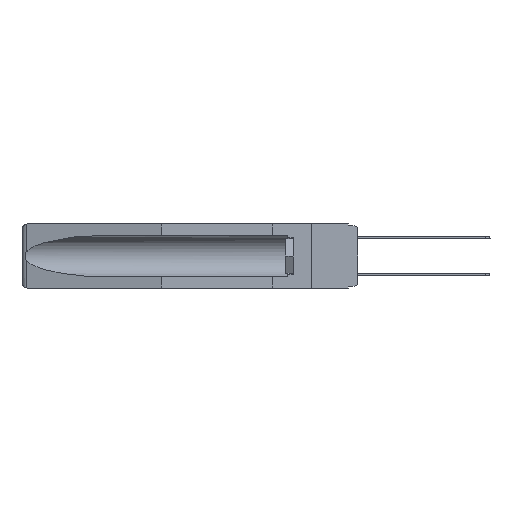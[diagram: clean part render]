
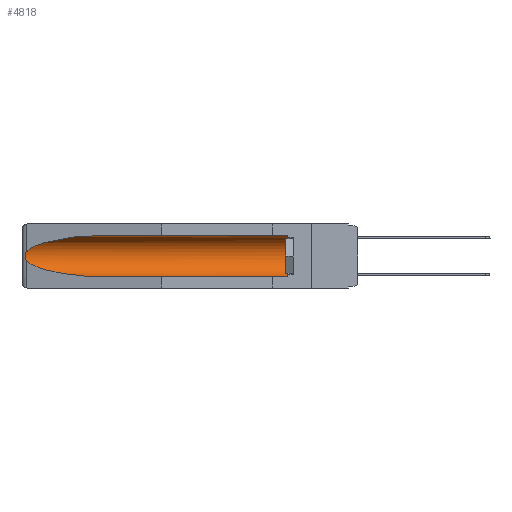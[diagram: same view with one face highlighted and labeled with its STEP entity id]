
A CAD part, left-side view. The second image highlights one B-rep face of the part: STEP entity #4818.
In plain terms, the highlighted cylindrical face has radius 2.857 mm (diameter 5.715 mm), a partial arc.
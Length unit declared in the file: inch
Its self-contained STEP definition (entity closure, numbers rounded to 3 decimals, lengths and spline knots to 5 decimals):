
#1000 = CIRCLE ( 'NONE', #1314, 0.1125 ) ;
#1314 = AXIS2_PLACEMENT_3D ( 'NONE', #4957, #11107, #17222 ) ;
#2257 = CARTESIAN_POINT ( 'NONE',  ( 0.26537, 1.52718, -0.14972 ) ) ;
#2545 = CARTESIAN_POINT ( 'NONE',  ( 0.155, 1.07973, -0.059 ) ) ;
#2866 = EDGE_LOOP ( 'NONE', ( #5129, #5025, #16525, #17286, #12545, #16399 ) ) ;
#3478 = CARTESIAN_POINT ( 'NONE',  ( 0.155, 0.126, -0.059 ) ) ;
#3984 = CARTESIAN_POINT ( 'NONE',  ( 0.26597, 1.52961, -0.15275 ) ) ;
#4110 = VERTEX_POINT ( 'NONE', #15546 ) ;
#4141 = CARTESIAN_POINT ( 'NONE',  ( 0.155, -0.30754, -0.059 ) ) ;
#4308 = CARTESIAN_POINT ( 'NONE',  ( 0.26537, 1.52718, -0.14972 ) ) ;
#4818 = ADVANCED_FACE ( 'NONE', ( #8857 ), #13596, .F. ) ;
#4957 = CARTESIAN_POINT ( 'NONE',  ( 0.155, 0.126, -0.1715 ) ) ;
#5025 = ORIENTED_EDGE ( 'NONE', *, *, #14688, .T. ) ;
#5129 = ORIENTED_EDGE ( 'NONE', *, *, #16868, .T. ) ;
#5577 = DIRECTION ( 'NONE',  ( 0., 1., 0. ) ) ;
#5591 = CARTESIAN_POINT ( 'NONE',  ( 0.2673, 1.5327, -0.16383 ) ) ;
#5662 = EDGE_CURVE ( 'NONE', #13260, #12399, #17645, .T. ) ;
#6002 =( BOUNDED_CURVE ( )  B_SPLINE_CURVE ( 3, ( #2545, #19328, #19225, #2257 ),
 .UNSPECIFIED., .F., .F. ) 
 B_SPLINE_CURVE_WITH_KNOTS ( ( 4, 4 ),
 ( 4.71239, 6.08839 ),
 .UNSPECIFIED. ) 
 CURVE ( )  GEOMETRIC_REPRESENTATION_ITEM ( )  RATIONAL_B_SPLINE_CURVE ( ( 1., 0.848, 0.848, 1. ) ) 
 REPRESENTATION_ITEM ( '' )  );
#6459 = VECTOR ( 'NONE', #8764, 39.37008 ) ;
#6905 = CARTESIAN_POINT ( 'NONE',  ( 0.155, 1.07973, -0.284 ) ) ;
#7449 = DIRECTION ( 'NONE',  ( 0., 1., 0. ) ) ;
#8235 = B_SPLINE_CURVE_WITH_KNOTS ( 'NONE', 3,
 ( #16258, #3984, #13250, #5591, #14642, #8413, #19362, #14544, #17466, #17764 ),
 .UNSPECIFIED., .F., .F.,
 ( 4, 2, 2, 2, 4 ),
 ( 0., 0.00029, 0.00058, 0.00087, 0.00117 ),
 .UNSPECIFIED. ) ;
#8413 = CARTESIAN_POINT ( 'NONE',  ( 0.2675, 1.53308, -0.17534 ) ) ;
#8764 = DIRECTION ( 'NONE',  ( 0., 1., 0. ) ) ;
#8857 = FACE_OUTER_BOUND ( 'NONE', #2866, .T. ) ;
#9173 = CARTESIAN_POINT ( 'NONE',  ( 0.26537, 1.52718, -0.19328 ) ) ;
#10456 = AXIS2_PLACEMENT_3D ( 'NONE', #11911, #7449, #18201 ) ;
#11107 = DIRECTION ( 'NONE',  ( 0., -1., 0. ) ) ;
#11263 = CARTESIAN_POINT ( 'NONE',  ( 0.21114, 1.30732, -0.284 ) ) ;
#11604 = VERTEX_POINT ( 'NONE', #9173 ) ;
#11829 = EDGE_CURVE ( 'NONE', #13260, #16306, #1000, .T. ) ;
#11847 = EDGE_CURVE ( 'NONE', #16306, #4110, #19413, .T. ) ;
#11911 = CARTESIAN_POINT ( 'NONE',  ( 0.155, -0.30754, -0.1715 ) ) ;
#12399 = VERTEX_POINT ( 'NONE', #14572 ) ;
#12412 = VECTOR ( 'NONE', #5577, 39.37008 ) ;
#12545 = ORIENTED_EDGE ( 'NONE', *, *, #11829, .T. ) ;
#12826 = EDGE_CURVE ( 'NONE', #11604, #12399, #14994, .T. ) ;
#13250 = CARTESIAN_POINT ( 'NONE',  ( 0.26654, 1.53092, -0.15636 ) ) ;
#13260 = VERTEX_POINT ( 'NONE', #15848 ) ;
#13596 = CYLINDRICAL_SURFACE ( 'NONE', #10456, 0.1125 ) ;
#14544 = CARTESIAN_POINT ( 'NONE',  ( 0.26655, 1.53094, -0.18657 ) ) ;
#14572 = CARTESIAN_POINT ( 'NONE',  ( 0.155, 1.07973, -0.284 ) ) ;
#14642 = CARTESIAN_POINT ( 'NONE',  ( 0.2675, 1.53308, -0.16763 ) ) ;
#14688 = EDGE_CURVE ( 'NONE', #19650, #11604, #8235, .T. ) ;
#14994 =( BOUNDED_CURVE ( )  B_SPLINE_CURVE ( 3, ( #19271, #16261, #11263, #6905 ),
 .UNSPECIFIED., .F., .F. ) 
 B_SPLINE_CURVE_WITH_KNOTS ( ( 4, 4 ),
 ( 0.1948, 1.5708 ),
 .UNSPECIFIED. ) 
 CURVE ( )  GEOMETRIC_REPRESENTATION_ITEM ( )  RATIONAL_B_SPLINE_CURVE ( ( 1., 0.848, 0.848, 1. ) ) 
 REPRESENTATION_ITEM ( '' )  );
#15546 = CARTESIAN_POINT ( 'NONE',  ( 0.155, 1.07973, -0.059 ) ) ;
#15848 = CARTESIAN_POINT ( 'NONE',  ( 0.155, 0.126, -0.284 ) ) ;
#16239 = CARTESIAN_POINT ( 'NONE',  ( 0.155, -0.30754, -0.284 ) ) ;
#16258 = CARTESIAN_POINT ( 'NONE',  ( 0.26537, 1.52718, -0.14972 ) ) ;
#16261 = CARTESIAN_POINT ( 'NONE',  ( 0.25451, 1.48313, -0.24835 ) ) ;
#16306 = VERTEX_POINT ( 'NONE', #3478 ) ;
#16399 = ORIENTED_EDGE ( 'NONE', *, *, #11847, .T. ) ;
#16525 = ORIENTED_EDGE ( 'NONE', *, *, #12826, .T. ) ;
#16868 = EDGE_CURVE ( 'NONE', #4110, #19650, #6002, .T. ) ;
#17222 = DIRECTION ( 'NONE',  ( 0., 0., 1. ) ) ;
#17286 = ORIENTED_EDGE ( 'NONE', *, *, #5662, .F. ) ;
#17466 = CARTESIAN_POINT ( 'NONE',  ( 0.26597, 1.5296, -0.19026 ) ) ;
#17645 = LINE ( 'NONE', #16239, #12412 ) ;
#17764 = CARTESIAN_POINT ( 'NONE',  ( 0.26537, 1.52718, -0.19328 ) ) ;
#18201 = DIRECTION ( 'NONE',  ( 0., 0., 1. ) ) ;
#19225 = CARTESIAN_POINT ( 'NONE',  ( 0.25451, 1.48313, -0.09465 ) ) ;
#19271 = CARTESIAN_POINT ( 'NONE',  ( 0.26537, 1.52718, -0.19328 ) ) ;
#19328 = CARTESIAN_POINT ( 'NONE',  ( 0.21114, 1.30732, -0.059 ) ) ;
#19362 = CARTESIAN_POINT ( 'NONE',  ( 0.2673, 1.53269, -0.17917 ) ) ;
#19413 = LINE ( 'NONE', #4141, #6459 ) ;
#19650 = VERTEX_POINT ( 'NONE', #4308 ) ;
